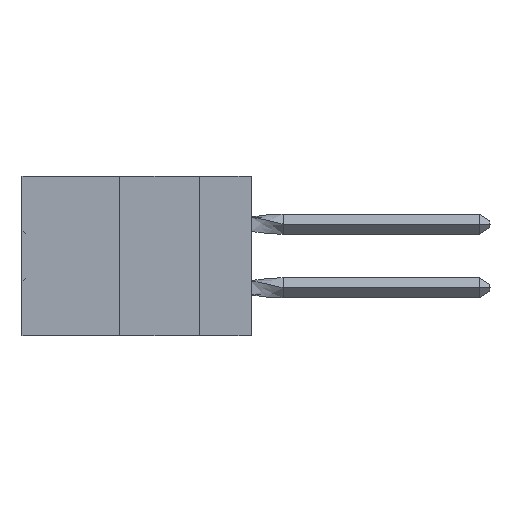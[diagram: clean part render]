
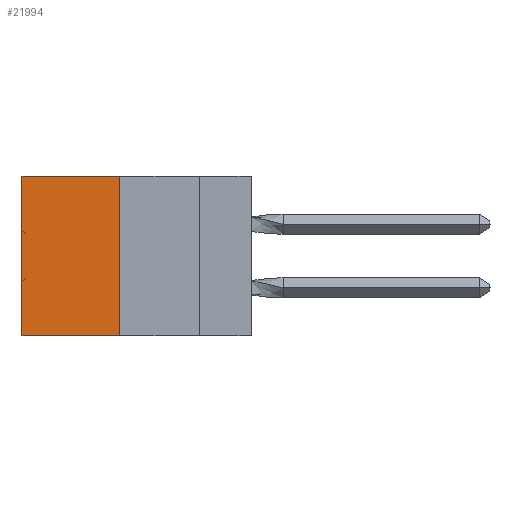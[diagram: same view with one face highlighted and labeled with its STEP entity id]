
A CAD part, left-side view. The second image highlights one B-rep face of the part: STEP entity #21994.
In plain terms, the highlighted planar face has unit normal (-1, 0, 0).
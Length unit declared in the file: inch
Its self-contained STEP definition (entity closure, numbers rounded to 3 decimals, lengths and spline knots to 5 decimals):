
#7167 = DIRECTION ( 'NONE',  ( 0., 0., -1. ) ) ;
#8096 = CARTESIAN_POINT ( 'NONE',  ( 0.305, 0.413, -0.5 ) ) ;
#10428 = EDGE_CURVE ( 'NONE', #40998, #37495, #54191, .T. ) ;
#11806 = VECTOR ( 'NONE', #39658, 39.37008 ) ;
#13705 = EDGE_CURVE ( 'NONE', #15986, #35266, #16728, .T. ) ;
#14482 = CARTESIAN_POINT ( 'NONE',  ( 0.305, 0.413, -0.5 ) ) ;
#14567 = ORIENTED_EDGE ( 'NONE', *, *, #13705, .T. ) ;
#15442 = DIRECTION ( 'NONE',  ( 0., 1., 0. ) ) ;
#15986 = VERTEX_POINT ( 'NONE', #53291 ) ;
#16522 = AXIS2_PLACEMENT_3D ( 'NONE', #8096, #51343, #57425 ) ;
#16728 = LINE ( 'NONE', #44408, #11806 ) ;
#18321 = LINE ( 'NONE', #14482, #57713 ) ;
#21485 = VECTOR ( 'NONE', #57805, 39.37008 ) ;
#21514 = EDGE_CURVE ( 'NONE', #37495, #35266, #18321, .T. ) ;
#21994 = ADVANCED_FACE ( 'NONE', ( #38688 ), #42376, .F. ) ;
#25275 = CARTESIAN_POINT ( 'NONE',  ( 0.305, 0.413, -0.5 ) ) ;
#28871 = VECTOR ( 'NONE', #7167, 39.37008 ) ;
#30531 = ORIENTED_EDGE ( 'NONE', *, *, #46268, .T. ) ;
#31602 = CARTESIAN_POINT ( 'NONE',  ( 0.305, 0.413, 0. ) ) ;
#35266 = VERTEX_POINT ( 'NONE', #53804 ) ;
#37495 = VERTEX_POINT ( 'NONE', #53859 ) ;
#38415 = LINE ( 'NONE', #40161, #21485 ) ;
#38688 = FACE_OUTER_BOUND ( 'NONE', #53333, .T. ) ;
#39658 = DIRECTION ( 'NONE',  ( 0., 0., -1. ) ) ;
#40161 = CARTESIAN_POINT ( 'NONE',  ( 0.305, 0.413, 0. ) ) ;
#40720 = ORIENTED_EDGE ( 'NONE', *, *, #10428, .F. ) ;
#40998 = VERTEX_POINT ( 'NONE', #31602 ) ;
#42376 = PLANE ( 'NONE',  #16522 ) ;
#44408 = CARTESIAN_POINT ( 'NONE',  ( 0.305, 0.72, -0.5 ) ) ;
#46268 = EDGE_CURVE ( 'NONE', #40998, #15986, #38415, .T. ) ;
#49388 = ORIENTED_EDGE ( 'NONE', *, *, #21514, .F. ) ;
#51343 = DIRECTION ( 'NONE',  ( 1., 0., 0. ) ) ;
#53291 = CARTESIAN_POINT ( 'NONE',  ( 0.305, 0.72, 0. ) ) ;
#53333 = EDGE_LOOP ( 'NONE', ( #14567, #49388, #40720, #30531 ) ) ;
#53804 = CARTESIAN_POINT ( 'NONE',  ( 0.305, 0.72, -0.5 ) ) ;
#53859 = CARTESIAN_POINT ( 'NONE',  ( 0.305, 0.413, -0.5 ) ) ;
#54191 = LINE ( 'NONE', #25275, #28871 ) ;
#57425 = DIRECTION ( 'NONE',  ( 0., 0., -1. ) ) ;
#57713 = VECTOR ( 'NONE', #15442, 39.37008 ) ;
#57805 = DIRECTION ( 'NONE',  ( 0., 1., 0. ) ) ;
